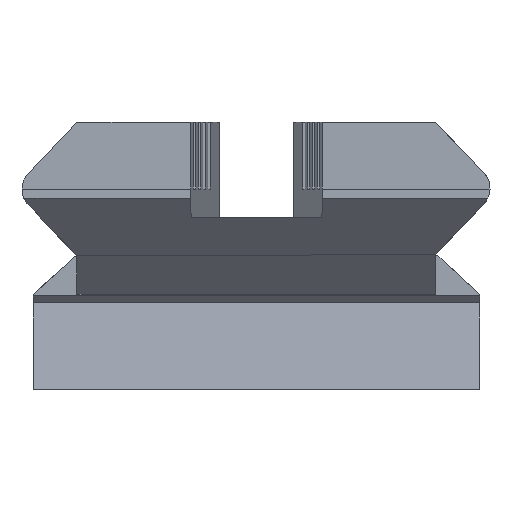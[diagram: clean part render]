
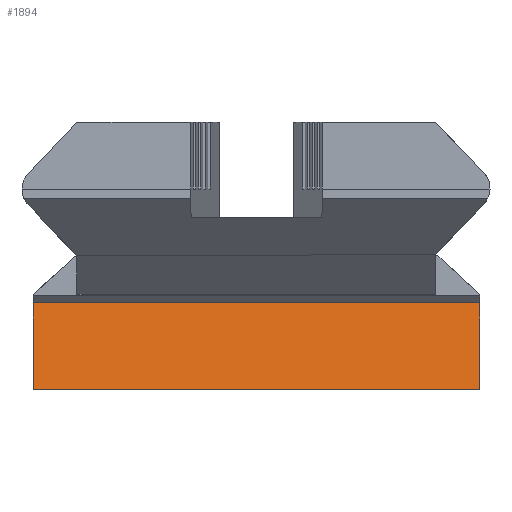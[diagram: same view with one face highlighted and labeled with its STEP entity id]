
A CAD part, front view. The second image highlights one B-rep face of the part: STEP entity #1894.
In plain terms, the highlighted planar face has unit normal (0, -0.987, 0.161).
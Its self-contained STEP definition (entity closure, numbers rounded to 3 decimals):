
#75=FACE_OUTER_BOUND('',#173,.T.);
#173=EDGE_LOOP('',(#1235,#1236,#1237,#1238));
#280=LINE('',#2699,#519);
#281=LINE('',#2702,#520);
#282=LINE('',#2704,#521);
#283=LINE('',#2705,#522);
#519=VECTOR('',#2161,10.);
#520=VECTOR('',#2164,10.);
#521=VECTOR('',#2165,10.);
#522=VECTOR('',#2166,10.);
#752=VERTEX_POINT('',#2686);
#758=VERTEX_POINT('',#2697);
#759=VERTEX_POINT('',#2701);
#760=VERTEX_POINT('',#2703);
#947=EDGE_CURVE('',#758,#752,#280,.T.);
#948=EDGE_CURVE('',#759,#752,#281,.T.);
#949=EDGE_CURVE('',#758,#760,#282,.T.);
#950=EDGE_CURVE('',#759,#760,#283,.T.);
#1235=ORIENTED_EDGE('',*,*,#948,.T.);
#1236=ORIENTED_EDGE('',*,*,#947,.F.);
#1237=ORIENTED_EDGE('',*,*,#949,.T.);
#1238=ORIENTED_EDGE('',*,*,#950,.F.);
#1803=PLANE('',#2006);
#1894=ADVANCED_FACE('',(#75),#1803,.F.);
#2006=AXIS2_PLACEMENT_3D('',#2700,#2162,#2163);
#2161=DIRECTION('',(0.,0.161,0.987));
#2162=DIRECTION('center_axis',(0.,0.987,-0.161));
#2163=DIRECTION('ref_axis',(0.,0.161,0.987));
#2164=DIRECTION('',(-1.,0.,0.));
#2165=DIRECTION('',(1.,0.,0.));
#2166=DIRECTION('',(0.,-0.161,-0.987));
#2686=CARTESIAN_POINT('',(-7.554,-8.392,3.8));
#2697=CARTESIAN_POINT('',(-7.554,-9.012,0.));
#2699=CARTESIAN_POINT('',(-7.554,-8.599,2.534));
#2700=CARTESIAN_POINT('Origin',(-7.554,-9.012,0.));
#2701=CARTESIAN_POINT('',(11.946,-8.392,3.8));
#2702=CARTESIAN_POINT('',(-7.554,-8.392,3.8));
#2703=CARTESIAN_POINT('',(11.946,-9.012,0.));
#2704=CARTESIAN_POINT('',(-7.554,-9.012,0.));
#2705=CARTESIAN_POINT('',(11.946,-9.012,0.));
